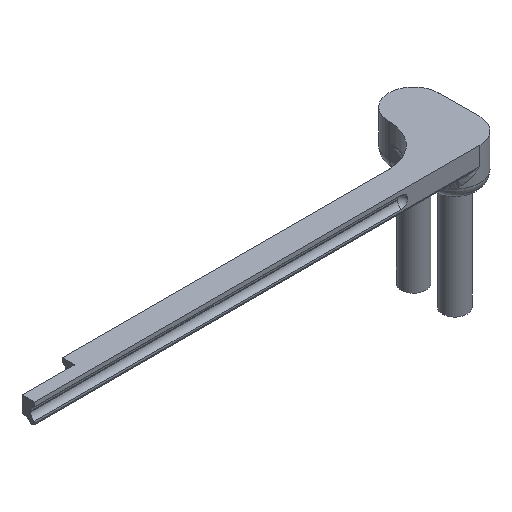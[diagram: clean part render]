
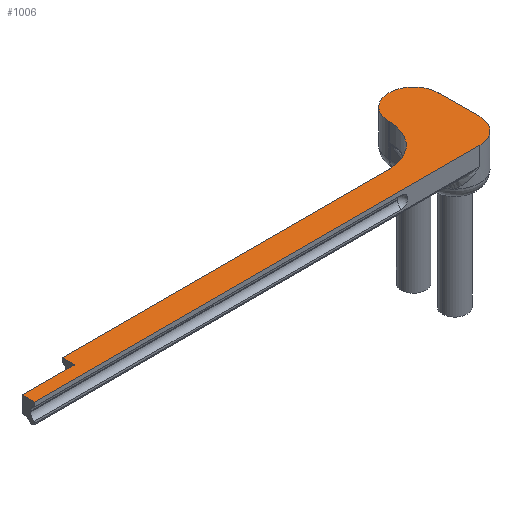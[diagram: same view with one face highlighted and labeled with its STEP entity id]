
A CAD part, isometric view. The second image highlights one B-rep face of the part: STEP entity #1006.
In plain terms, the highlighted planar face has unit normal (0, 0, 1).
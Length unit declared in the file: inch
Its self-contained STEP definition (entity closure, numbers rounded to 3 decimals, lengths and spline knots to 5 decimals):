
#30 = EDGE_CURVE ( 'NONE', #68, #1440, #703, .T. ) ;
#33 = EDGE_CURVE ( 'NONE', #68, #1522, #1060, .T. ) ;
#46 = EDGE_CURVE ( 'NONE', #1522, #601, #1734, .T. ) ;
#58 = EDGE_CURVE ( 'NONE', #601, #819, #1019, .T. ) ;
#61 = CARTESIAN_POINT ( 'NONE',  ( 2.0528, -0.59002, 0.19685 ) ) ;
#63 = EDGE_CURVE ( 'NONE', #1479, #296, #984, .T. ) ;
#68 = VERTEX_POINT ( 'NONE', #390 ) ;
#76 = EDGE_CURVE ( 'NONE', #296, #541, #597, .T. ) ;
#86 = EDGE_CURVE ( 'NONE', #541, #603, #934, .T. ) ;
#94 = EDGE_CURVE ( 'NONE', #603, #868, #144, .T. ) ;
#109 = EDGE_CURVE ( 'NONE', #868, #1440, #1598, .T. ) ;
#111 = DIRECTION ( 'NONE',  ( 0., 0., 1. ) ) ;
#144 = LINE ( 'NONE', #1241, #1238 ) ;
#167 = ORIENTED_EDGE ( 'NONE', *, *, #46, .T. ) ;
#195 = VECTOR ( 'NONE', #850, 39.37008 ) ;
#224 = DIRECTION ( 'NONE',  ( 1., 0., 0. ) ) ;
#234 = DIRECTION ( 'NONE',  ( 1., 0., 0. ) ) ;
#240 = CARTESIAN_POINT ( 'NONE',  ( 2.0528, 0., 0.19685 ) ) ;
#244 = DIRECTION ( 'NONE',  ( 0., 0., 1. ) ) ;
#270 = ORIENTED_EDGE ( 'NONE', *, *, #30, .F. ) ;
#294 = LINE ( 'NONE', #359, #397 ) ;
#295 = VECTOR ( 'NONE', #234, 39.37008 ) ;
#296 = VERTEX_POINT ( 'NONE', #960 ) ;
#359 = CARTESIAN_POINT ( 'NONE',  ( 0., -0.59002, 0.19685 ) ) ;
#371 = CIRCLE ( 'NONE', #767, 0.23901 ) ;
#383 = CARTESIAN_POINT ( 'NONE',  ( 6.31381, -0.59002, 0.19685 ) ) ;
#390 = CARTESIAN_POINT ( 'NONE',  ( 2.5528, -0.3538, 0.19685 ) ) ;
#396 = DIRECTION ( 'NONE',  ( 0., -1., 0. ) ) ;
#397 = VECTOR ( 'NONE', #224, 39.37008 ) ;
#405 = DIRECTION ( 'NONE',  ( 0., -1., 0. ) ) ;
#420 = ORIENTED_EDGE ( 'NONE', *, *, #33, .T. ) ;
#440 = AXIS2_PLACEMENT_3D ( 'NONE', #1249, #111, #1116 ) ;
#539 = EDGE_CURVE ( 'NONE', #819, #543, #294, .T. ) ;
#541 = VERTEX_POINT ( 'NONE', #943 ) ;
#543 = VERTEX_POINT ( 'NONE', #383 ) ;
#545 = CARTESIAN_POINT ( 'NONE',  ( 2.5528, 0., 0.19685 ) ) ;
#597 = LINE ( 'NONE', #1643, #195 ) ;
#601 = VERTEX_POINT ( 'NONE', #1453 ) ;
#603 = VERTEX_POINT ( 'NONE', #636 ) ;
#615 = CARTESIAN_POINT ( 'NONE',  ( 5.68389, 0.0399, 0.19685 ) ) ;
#636 = CARTESIAN_POINT ( 'NONE',  ( 6.07759, 0.04269, 0.19685 ) ) ;
#656 = VECTOR ( 'NONE', #1368, 39.37008 ) ;
#703 = LINE ( 'NONE', #1498, #295 ) ;
#745 = ORIENTED_EDGE ( 'NONE', *, *, #109, .T. ) ;
#756 = DIRECTION ( 'NONE',  ( 1., 0., 0. ) ) ;
#767 = AXIS2_PLACEMENT_3D ( 'NONE', #1613, #825, #1769 ) ;
#768 = DIRECTION ( 'NONE',  ( -1., 0., 0. ) ) ;
#785 = EDGE_CURVE ( 'NONE', #543, #1479, #371, .T. ) ;
#819 = VERTEX_POINT ( 'NONE', #61 ) ;
#825 = DIRECTION ( 'NONE',  ( 0., 0., 1. ) ) ;
#846 = AXIS2_PLACEMENT_3D ( 'NONE', #615, #1565, #768 ) ;
#850 = DIRECTION ( 'NONE',  ( -0.007, 1., 0. ) ) ;
#868 = VERTEX_POINT ( 'NONE', #981 ) ;
#934 = CIRCLE ( 'NONE', #969, 0.23622 ) ;
#943 = CARTESIAN_POINT ( 'NONE',  ( 6.55004, 0.04269, 0.19685 ) ) ;
#947 = ORIENTED_EDGE ( 'NONE', *, *, #58, .T. ) ;
#960 = CARTESIAN_POINT ( 'NONE',  ( 6.5528, -0.34762, 0.19685 ) ) ;
#969 = AXIS2_PLACEMENT_3D ( 'NONE', #1694, #1590, #756 ) ;
#971 = DIRECTION ( 'NONE',  ( 0., -1., 0. ) ) ;
#981 = CARTESIAN_POINT ( 'NONE',  ( 6.07759, 0.0399, 0.19685 ) ) ;
#984 = CIRCLE ( 'NONE', #990, 0.23901 ) ;
#990 = AXIS2_PLACEMENT_3D ( 'NONE', #1102, #244, #1237 ) ;
#995 = ORIENTED_EDGE ( 'NONE', *, *, #539, .T. ) ;
#1006 = ADVANCED_FACE ( 'NONE', ( #1355 ), #1654, .T. ) ;
#1019 = LINE ( 'NONE', #240, #1686 ) ;
#1060 = LINE ( 'NONE', #545, #1381 ) ;
#1097 = CARTESIAN_POINT ( 'NONE',  ( 6.55283, -0.35101, 0.19685 ) ) ;
#1102 = CARTESIAN_POINT ( 'NONE',  ( 6.31381, -0.35101, 0.19685 ) ) ;
#1116 = DIRECTION ( 'NONE',  ( 1., 0., 0. ) ) ;
#1233 = CARTESIAN_POINT ( 'NONE',  ( 0., -0.46882, 0.19685 ) ) ;
#1237 = DIRECTION ( 'NONE',  ( 1., 0., 0. ) ) ;
#1238 = VECTOR ( 'NONE', #405, 39.37008 ) ;
#1241 = CARTESIAN_POINT ( 'NONE',  ( 6.07759, 0.04269, 0.19685 ) ) ;
#1249 = CARTESIAN_POINT ( 'NONE',  ( 0., 0., 0.19685 ) ) ;
#1290 = ORIENTED_EDGE ( 'NONE', *, *, #86, .T. ) ;
#1322 = ORIENTED_EDGE ( 'NONE', *, *, #785, .T. ) ;
#1355 = FACE_OUTER_BOUND ( 'NONE', #1629, .T. ) ;
#1368 = DIRECTION ( 'NONE',  ( -1., 0., 0. ) ) ;
#1381 = VECTOR ( 'NONE', #971, 39.37008 ) ;
#1440 = VERTEX_POINT ( 'NONE', #1765 ) ;
#1453 = CARTESIAN_POINT ( 'NONE',  ( 2.0528, -0.46882, 0.19685 ) ) ;
#1479 = VERTEX_POINT ( 'NONE', #1097 ) ;
#1498 = CARTESIAN_POINT ( 'NONE',  ( 0., -0.3538, 0.19685 ) ) ;
#1522 = VERTEX_POINT ( 'NONE', #1664 ) ;
#1555 = ORIENTED_EDGE ( 'NONE', *, *, #76, .T. ) ;
#1565 = DIRECTION ( 'NONE',  ( 0., 0., -1. ) ) ;
#1587 = ORIENTED_EDGE ( 'NONE', *, *, #63, .T. ) ;
#1590 = DIRECTION ( 'NONE',  ( 0., 0., 1. ) ) ;
#1598 = CIRCLE ( 'NONE', #846, 0.3937 ) ;
#1613 = CARTESIAN_POINT ( 'NONE',  ( 6.31381, -0.35101, 0.19685 ) ) ;
#1629 = EDGE_LOOP ( 'NONE', ( #270, #420, #167, #947, #995, #1322, #1587, #1555, #1290, #1789, #745 ) ) ;
#1643 = CARTESIAN_POINT ( 'NONE',  ( 6.55004, 0.04269, 0.19685 ) ) ;
#1654 = PLANE ( 'NONE',  #440 ) ;
#1664 = CARTESIAN_POINT ( 'NONE',  ( 2.5528, -0.46882, 0.19685 ) ) ;
#1686 = VECTOR ( 'NONE', #396, 39.37008 ) ;
#1694 = CARTESIAN_POINT ( 'NONE',  ( 6.31381, 0.04269, 0.19685 ) ) ;
#1734 = LINE ( 'NONE', #1233, #656 ) ;
#1765 = CARTESIAN_POINT ( 'NONE',  ( 5.68389, -0.3538, 0.19685 ) ) ;
#1769 = DIRECTION ( 'NONE',  ( 1., 0., 0. ) ) ;
#1789 = ORIENTED_EDGE ( 'NONE', *, *, #94, .T. ) ;
